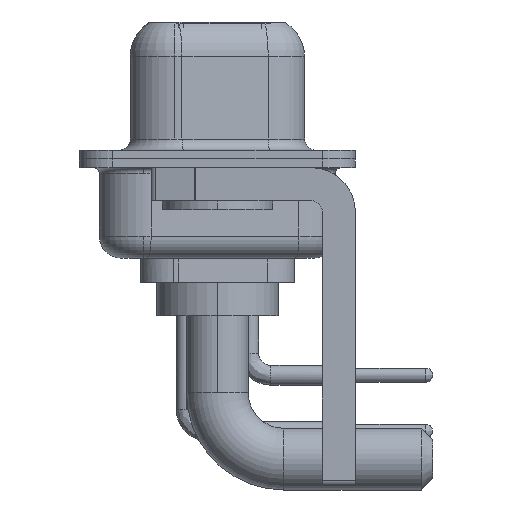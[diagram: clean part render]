
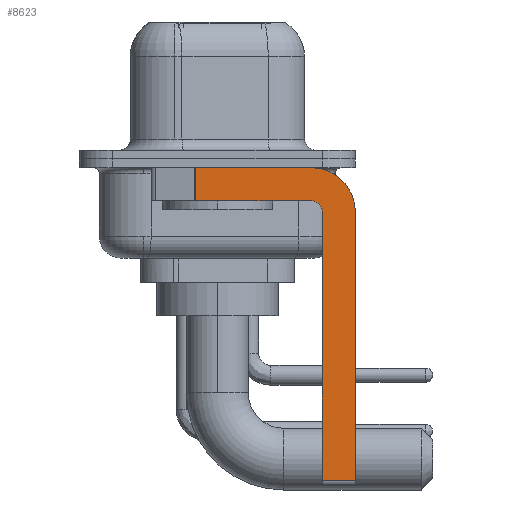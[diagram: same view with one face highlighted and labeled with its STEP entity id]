
A CAD part, left-side view. The second image highlights one B-rep face of the part: STEP entity #8623.
In plain terms, the highlighted planar face has unit normal (-1, 0, 0).
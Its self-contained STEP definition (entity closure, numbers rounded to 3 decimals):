
#114 = CARTESIAN_POINT ( 'NONE',  ( -2.9, -4.75, -2.4 ) ) ;
#370 = CARTESIAN_POINT ( 'NONE',  ( -2.9, 0.978, -0.4 ) ) ;
#1188 = ORIENTED_EDGE ( 'NONE', *, *, #9972, .F. ) ;
#1548 = CARTESIAN_POINT ( 'NONE',  ( -2.9, 3., -0.4 ) ) ;
#1773 = FACE_OUTER_BOUND ( 'NONE', #18182, .T. ) ;
#1872 = DIRECTION ( 'NONE',  ( 1., 0., 0. ) ) ;
#1985 = DIRECTION ( 'NONE',  ( 0., 0., -1. ) ) ;
#2124 = LINE ( 'NONE', #16775, #19718 ) ;
#2735 = EDGE_CURVE ( 'NONE', #18030, #10786, #6783, .T. ) ;
#3064 = CARTESIAN_POINT ( 'NONE',  ( -2.9, -6.25, -2.4 ) ) ;
#3501 = CARTESIAN_POINT ( 'NONE',  ( -2.9, -4.25, -2.4 ) ) ;
#3593 = CARTESIAN_POINT ( 'NONE',  ( -2.9, -4.75, -14.8 ) ) ;
#3632 = ORIENTED_EDGE ( 'NONE', *, *, #11778, .T. ) ;
#3879 = CARTESIAN_POINT ( 'NONE',  ( -2.9, -6.25, -14.55 ) ) ;
#4053 = ORIENTED_EDGE ( 'NONE', *, *, #13976, .T. ) ;
#4981 = ORIENTED_EDGE ( 'NONE', *, *, #11197, .F. ) ;
#4991 = DIRECTION ( 'NONE',  ( 1., 0., 0. ) ) ;
#5073 = PLANE ( 'NONE',  #15791 ) ;
#6242 = LINE ( 'NONE', #11202, #17190 ) ;
#6740 = EDGE_CURVE ( 'NONE', #8756, #10650, #17774, .T. ) ;
#6779 = VECTOR ( 'NONE', #7085, 1000. ) ;
#6783 = LINE ( 'NONE', #8257, #19422 ) ;
#6949 = CARTESIAN_POINT ( 'NONE',  ( -2.9, -4.75, -14.55 ) ) ;
#7085 = DIRECTION ( 'NONE',  ( 0., 0., 1. ) ) ;
#7391 = CARTESIAN_POINT ( 'NONE',  ( -2.9, -4.25, -0.4 ) ) ;
#8057 = AXIS2_PLACEMENT_3D ( 'NONE', #10875, #20656, #14177 ) ;
#8233 = CARTESIAN_POINT ( 'NONE',  ( -2.9, -4.25, -2.4 ) ) ;
#8257 = CARTESIAN_POINT ( 'NONE',  ( -2.9, -4.25, -1.9 ) ) ;
#8587 = DIRECTION ( 'NONE',  ( 0., 0., -1. ) ) ;
#8623 = ADVANCED_FACE ( 'NONE', ( #1773 ), #5073, .F. ) ;
#8756 = VERTEX_POINT ( 'NONE', #7391 ) ;
#9972 = EDGE_CURVE ( 'NONE', #12660, #16649, #13547, .T. ) ;
#10067 = DIRECTION ( 'NONE',  ( 0., 0., -1. ) ) ;
#10650 = VERTEX_POINT ( 'NONE', #3064 ) ;
#10786 = VERTEX_POINT ( 'NONE', #16121 ) ;
#10875 = CARTESIAN_POINT ( 'NONE',  ( -2.9, -4.25, -2.4 ) ) ;
#11197 = EDGE_CURVE ( 'NONE', #10650, #15560, #15678, .T. ) ;
#11202 = CARTESIAN_POINT ( 'NONE',  ( -2.9, -4.25, -14.55 ) ) ;
#11778 = EDGE_CURVE ( 'NONE', #12631, #10786, #2124, .T. ) ;
#12631 = VERTEX_POINT ( 'NONE', #370 ) ;
#12660 = VERTEX_POINT ( 'NONE', #6949 ) ;
#13547 = LINE ( 'NONE', #3593, #6779 ) ;
#13870 = VECTOR ( 'NONE', #17910, 1000. ) ;
#13976 = EDGE_CURVE ( 'NONE', #12660, #15560, #6242, .T. ) ;
#14023 = AXIS2_PLACEMENT_3D ( 'NONE', #3501, #4991, #10067 ) ;
#14177 = DIRECTION ( 'NONE',  ( 0., 0., 1. ) ) ;
#14178 = DIRECTION ( 'NONE',  ( 0., 0., -1. ) ) ;
#14286 = CARTESIAN_POINT ( 'NONE',  ( -2.9, -6.25, -2.4 ) ) ;
#14398 = LINE ( 'NONE', #1548, #13870 ) ;
#14694 = EDGE_CURVE ( 'NONE', #16649, #18030, #17227, .T. ) ;
#15560 = VERTEX_POINT ( 'NONE', #3879 ) ;
#15678 = LINE ( 'NONE', #14286, #18352 ) ;
#15791 = AXIS2_PLACEMENT_3D ( 'NONE', #8233, #1872, #1985 ) ;
#16121 = CARTESIAN_POINT ( 'NONE',  ( -2.9, 0.978, -1.9 ) ) ;
#16191 = EDGE_CURVE ( 'NONE', #12631, #8756, #14398, .T. ) ;
#16649 = VERTEX_POINT ( 'NONE', #114 ) ;
#16775 = CARTESIAN_POINT ( 'NONE',  ( -2.9, 0.978, -1.9 ) ) ;
#17190 = VECTOR ( 'NONE', #19184, 1000. ) ;
#17227 = CIRCLE ( 'NONE', #8057, 0.5 ) ;
#17774 = CIRCLE ( 'NONE', #14023, 2. ) ;
#17910 = DIRECTION ( 'NONE',  ( 0., -1., 0. ) ) ;
#17951 = DIRECTION ( 'NONE',  ( 0., 1., 0. ) ) ;
#18030 = VERTEX_POINT ( 'NONE', #19090 ) ;
#18083 = ORIENTED_EDGE ( 'NONE', *, *, #14694, .F. ) ;
#18182 = EDGE_LOOP ( 'NONE', ( #19872, #3632, #18841, #18083, #1188, #4053, #4981, #19349 ) ) ;
#18352 = VECTOR ( 'NONE', #14178, 1000. ) ;
#18841 = ORIENTED_EDGE ( 'NONE', *, *, #2735, .F. ) ;
#19090 = CARTESIAN_POINT ( 'NONE',  ( -2.9, -4.25, -1.9 ) ) ;
#19184 = DIRECTION ( 'NONE',  ( 0., -1., 0. ) ) ;
#19349 = ORIENTED_EDGE ( 'NONE', *, *, #6740, .F. ) ;
#19422 = VECTOR ( 'NONE', #17951, 1000. ) ;
#19718 = VECTOR ( 'NONE', #8587, 1000. ) ;
#19872 = ORIENTED_EDGE ( 'NONE', *, *, #16191, .F. ) ;
#20656 = DIRECTION ( 'NONE',  ( -1., 0., 0. ) ) ;
